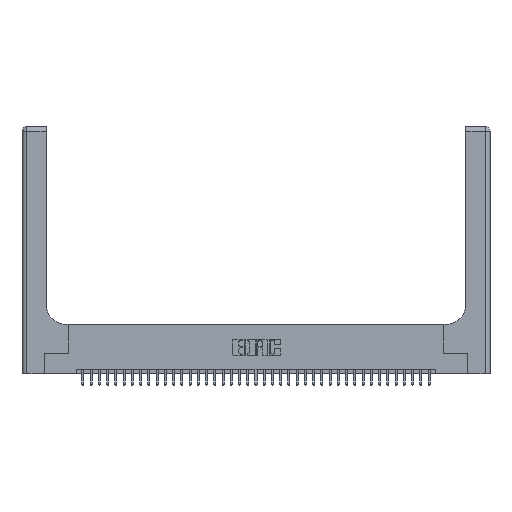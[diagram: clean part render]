
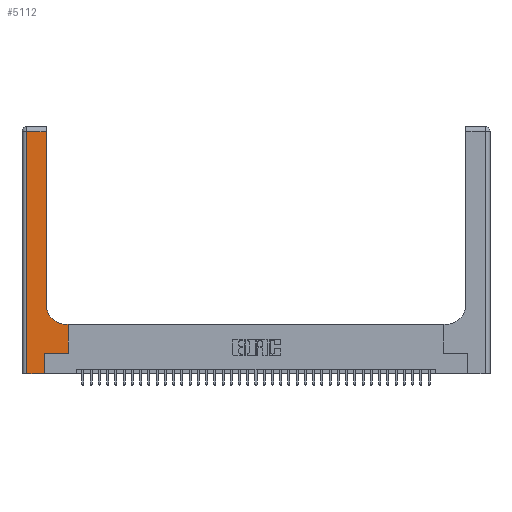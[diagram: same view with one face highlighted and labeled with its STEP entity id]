
A CAD part, top view. The second image highlights one B-rep face of the part: STEP entity #5112.
In plain terms, the highlighted planar face has unit normal (0, 0, 1).
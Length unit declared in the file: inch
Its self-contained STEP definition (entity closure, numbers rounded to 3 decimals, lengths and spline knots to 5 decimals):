
#99 = VECTOR ( 'NONE', #3716, 39.37008 ) ;
#1308 = VERTEX_POINT ( 'NONE', #11613 ) ;
#1449 = ORIENTED_EDGE ( 'NONE', *, *, #6631, .T. ) ;
#1885 = DIRECTION ( 'NONE',  ( 0., 0., -1. ) ) ;
#3065 = CARTESIAN_POINT ( 'NONE',  ( 0.269, 0., 0.37 ) ) ;
#3716 = DIRECTION ( 'NONE',  ( 1., 0., 0. ) ) ;
#3813 = EDGE_CURVE ( 'NONE', #19377, #19579, #28190, .T. ) ;
#3942 = EDGE_LOOP ( 'NONE', ( #33667, #29114, #26735, #10916, #37607, #36659, #1449, #5998, #19678 ) ) ;
#4169 = DIRECTION ( 'NONE',  ( 0., 1., 0. ) ) ;
#4296 = DIRECTION ( 'NONE',  ( 0., 1., 0. ) ) ;
#4556 = CARTESIAN_POINT ( 'NONE',  ( 0.5585, 0.25, 0.37 ) ) ;
#5072 = DIRECTION ( 'NONE',  ( 1., 0., 0. ) ) ;
#5112 = ADVANCED_FACE ( 'NONE', ( #11731 ), #16730, .F. ) ;
#5212 = VERTEX_POINT ( 'NONE', #29353 ) ;
#5829 = LINE ( 'NONE', #4556, #23600 ) ;
#5857 = DIRECTION ( 'NONE',  ( 0., 1., 0. ) ) ;
#5998 = ORIENTED_EDGE ( 'NONE', *, *, #38460, .T. ) ;
#6350 = VERTEX_POINT ( 'NONE', #31585 ) ;
#6631 = EDGE_CURVE ( 'NONE', #25788, #6350, #5829, .T. ) ;
#6976 = CARTESIAN_POINT ( 'NONE',  ( 0.06, 3., 0.37 ) ) ;
#8218 = VECTOR ( 'NONE', #4296, 39.37008 ) ;
#8561 = DIRECTION ( 'NONE',  ( 0., 0., -1. ) ) ;
#8586 = EDGE_CURVE ( 'NONE', #5212, #19377, #29066, .T. ) ;
#9780 = DIRECTION ( 'NONE',  ( -1., 0., 0. ) ) ;
#10915 = VECTOR ( 'NONE', #9780, 39.37008 ) ;
#10916 = ORIENTED_EDGE ( 'NONE', *, *, #25720, .T. ) ;
#11613 = CARTESIAN_POINT ( 'NONE',  ( 0.06, 0., 0.37 ) ) ;
#11731 = FACE_OUTER_BOUND ( 'NONE', #3942, .T. ) ;
#13620 = VERTEX_POINT ( 'NONE', #3065 ) ;
#15304 = LINE ( 'NONE', #19737, #22331 ) ;
#16125 = LINE ( 'NONE', #28601, #8218 ) ;
#16193 = CARTESIAN_POINT ( 'NONE',  ( 0.5415, 0.6, 0.37 ) ) ;
#16730 = PLANE ( 'NONE',  #17278 ) ;
#17163 = EDGE_CURVE ( 'NONE', #19579, #1308, #29644, .T. ) ;
#17278 = AXIS2_PLACEMENT_3D ( 'NONE', #18141, #8561, #38815 ) ;
#18141 = CARTESIAN_POINT ( 'NONE',  ( 0., 3., 0.37 ) ) ;
#18975 = DIRECTION ( 'NONE',  ( 0., -1., 0. ) ) ;
#19377 = VERTEX_POINT ( 'NONE', #29245 ) ;
#19579 = VERTEX_POINT ( 'NONE', #21611 ) ;
#19678 = ORIENTED_EDGE ( 'NONE', *, *, #31902, .T. ) ;
#19737 = CARTESIAN_POINT ( 'NONE',  ( 0., 0., 0.37 ) ) ;
#19777 = LINE ( 'NONE', #36811, #99 ) ;
#20823 = CIRCLE ( 'NONE', #31856, 0.25 ) ;
#21611 = CARTESIAN_POINT ( 'NONE',  ( 0.06, 2.94, 0.37 ) ) ;
#21715 = CARTESIAN_POINT ( 'NONE',  ( 0.2915, 0.6, 0.37 ) ) ;
#21961 = DIRECTION ( 'NONE',  ( -1., 0., 0. ) ) ;
#22331 = VECTOR ( 'NONE', #32039, 39.37008 ) ;
#22832 = CARTESIAN_POINT ( 'NONE',  ( 0.2915, 3., 0.37 ) ) ;
#23272 = VERTEX_POINT ( 'NONE', #28423 ) ;
#23600 = VECTOR ( 'NONE', #4169, 39.37008 ) ;
#23939 = VECTOR ( 'NONE', #5857, 39.37008 ) ;
#24067 = LINE ( 'NONE', #21715, #10915 ) ;
#25497 = VERTEX_POINT ( 'NONE', #16193 ) ;
#25720 = EDGE_CURVE ( 'NONE', #1308, #13620, #15304, .T. ) ;
#25788 = VERTEX_POINT ( 'NONE', #26387 ) ;
#26387 = CARTESIAN_POINT ( 'NONE',  ( 0.5585, 0.25, 0.37 ) ) ;
#26735 = ORIENTED_EDGE ( 'NONE', *, *, #17163, .T. ) ;
#26780 = VECTOR ( 'NONE', #18975, 39.37008 ) ;
#27846 = CARTESIAN_POINT ( 'NONE',  ( 0., 2.94, 0.37 ) ) ;
#28190 = LINE ( 'NONE', #27846, #31504 ) ;
#28423 = CARTESIAN_POINT ( 'NONE',  ( 0.269, 0.25, 0.37 ) ) ;
#28601 = CARTESIAN_POINT ( 'NONE',  ( 0.269, 0., 0.37 ) ) ;
#28797 = EDGE_CURVE ( 'NONE', #23272, #25788, #19777, .T. ) ;
#29066 = LINE ( 'NONE', #22832, #23939 ) ;
#29114 = ORIENTED_EDGE ( 'NONE', *, *, #3813, .T. ) ;
#29245 = CARTESIAN_POINT ( 'NONE',  ( 0.2915, 2.94, 0.37 ) ) ;
#29353 = CARTESIAN_POINT ( 'NONE',  ( 0.2915, 0.85, 0.37 ) ) ;
#29644 = LINE ( 'NONE', #6976, #26780 ) ;
#31504 = VECTOR ( 'NONE', #21961, 39.37008 ) ;
#31585 = CARTESIAN_POINT ( 'NONE',  ( 0.5585, 0.6, 0.37 ) ) ;
#31771 = EDGE_CURVE ( 'NONE', #13620, #23272, #16125, .T. ) ;
#31856 = AXIS2_PLACEMENT_3D ( 'NONE', #37775, #1885, #5072 ) ;
#31902 = EDGE_CURVE ( 'NONE', #25497, #5212, #20823, .T. ) ;
#32039 = DIRECTION ( 'NONE',  ( 1., 0., 0. ) ) ;
#33667 = ORIENTED_EDGE ( 'NONE', *, *, #8586, .T. ) ;
#36659 = ORIENTED_EDGE ( 'NONE', *, *, #28797, .T. ) ;
#36811 = CARTESIAN_POINT ( 'NONE',  ( 0.269, 0.25, 0.37 ) ) ;
#37607 = ORIENTED_EDGE ( 'NONE', *, *, #31771, .T. ) ;
#37775 = CARTESIAN_POINT ( 'NONE',  ( 0.5415, 0.85, 0.37 ) ) ;
#38460 = EDGE_CURVE ( 'NONE', #6350, #25497, #24067, .T. ) ;
#38815 = DIRECTION ( 'NONE',  ( -1., 0., 0. ) ) ;
